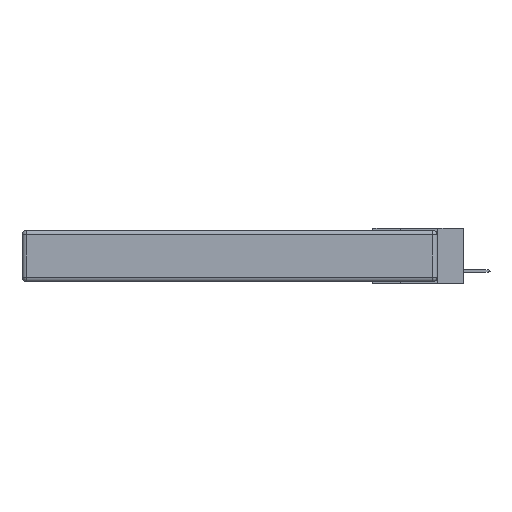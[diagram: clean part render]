
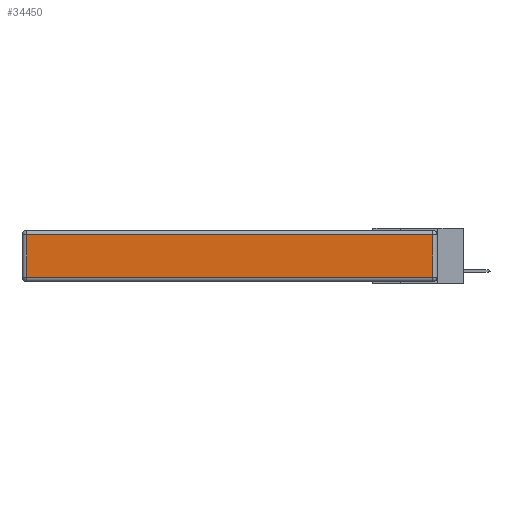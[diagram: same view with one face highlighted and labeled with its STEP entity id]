
A CAD part, left-side view. The second image highlights one B-rep face of the part: STEP entity #34450.
In plain terms, the highlighted planar face has unit normal (-1, 0, 0).
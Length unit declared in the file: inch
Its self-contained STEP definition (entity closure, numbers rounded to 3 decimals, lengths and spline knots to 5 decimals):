
#368 = EDGE_CURVE ( 'NONE', #8563, #32982, #14602, .T. ) ;
#820 = DIRECTION ( 'NONE',  ( 0., -1., 0. ) ) ;
#890 = EDGE_LOOP ( 'NONE', ( #22837, #4281, #29862, #5200 ) ) ;
#1604 = CARTESIAN_POINT ( 'NONE',  ( 0., 2.72, -0.343 ) ) ;
#3140 = LINE ( 'NONE', #1604, #28814 ) ;
#4281 = ORIENTED_EDGE ( 'NONE', *, *, #368, .T. ) ;
#4421 = DIRECTION ( 'NONE',  ( 0., 0., -1. ) ) ;
#4544 = VERTEX_POINT ( 'NONE', #29221 ) ;
#5200 = ORIENTED_EDGE ( 'NONE', *, *, #21112, .T. ) ;
#5263 = VECTOR ( 'NONE', #820, 39.37008 ) ;
#5523 = CARTESIAN_POINT ( 'NONE',  ( 0., 0.03, -0.343 ) ) ;
#5554 = CARTESIAN_POINT ( 'NONE',  ( 0., 2.75, -0.03 ) ) ;
#5830 = FACE_OUTER_BOUND ( 'NONE', #890, .T. ) ;
#5893 = CARTESIAN_POINT ( 'NONE',  ( 0., 0., -0.313 ) ) ;
#7739 = CARTESIAN_POINT ( 'NONE',  ( 0., 2.72, -0.03 ) ) ;
#7963 = LINE ( 'NONE', #5554, #14241 ) ;
#8563 = VERTEX_POINT ( 'NONE', #18085 ) ;
#11250 = VECTOR ( 'NONE', #24363, 39.37008 ) ;
#13749 = DIRECTION ( 'NONE',  ( 0., 1., 0. ) ) ;
#14241 = VECTOR ( 'NONE', #13749, 39.37008 ) ;
#14602 = LINE ( 'NONE', #5523, #11250 ) ;
#17097 = PLANE ( 'NONE',  #31411 ) ;
#17207 = DIRECTION ( 'NONE',  ( -1., 0., 0. ) ) ;
#17838 = LINE ( 'NONE', #5893, #5263 ) ;
#18085 = CARTESIAN_POINT ( 'NONE',  ( 0., 0.03, -0.313 ) ) ;
#18892 = EDGE_CURVE ( 'NONE', #32982, #19292, #7963, .T. ) ;
#19292 = VERTEX_POINT ( 'NONE', #7739 ) ;
#20917 = EDGE_CURVE ( 'NONE', #4544, #8563, #17838, .T. ) ;
#21112 = EDGE_CURVE ( 'NONE', #19292, #4544, #3140, .T. ) ;
#22837 = ORIENTED_EDGE ( 'NONE', *, *, #20917, .T. ) ;
#22923 = CARTESIAN_POINT ( 'NONE',  ( 0., 0., -0.343 ) ) ;
#24363 = DIRECTION ( 'NONE',  ( 0., 0., 1. ) ) ;
#27111 = CARTESIAN_POINT ( 'NONE',  ( 0., 0.03, -0.03 ) ) ;
#28814 = VECTOR ( 'NONE', #4421, 39.37008 ) ;
#29221 = CARTESIAN_POINT ( 'NONE',  ( 0., 2.72, -0.313 ) ) ;
#29862 = ORIENTED_EDGE ( 'NONE', *, *, #18892, .T. ) ;
#31411 = AXIS2_PLACEMENT_3D ( 'NONE', #22923, #17207, #33530 ) ;
#32982 = VERTEX_POINT ( 'NONE', #27111 ) ;
#33530 = DIRECTION ( 'NONE',  ( 0., 0., 1. ) ) ;
#34450 = ADVANCED_FACE ( 'NONE', ( #5830 ), #17097, .T. ) ;
